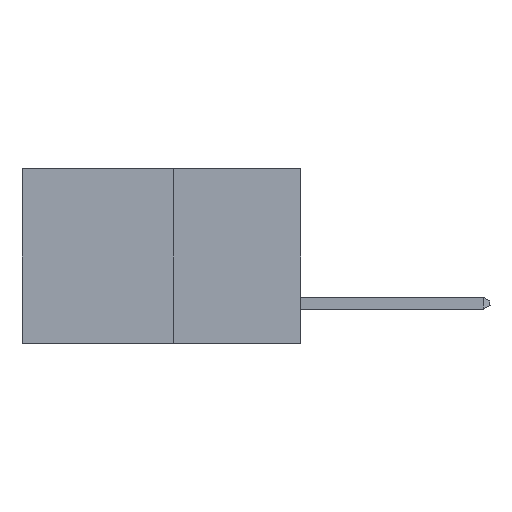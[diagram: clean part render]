
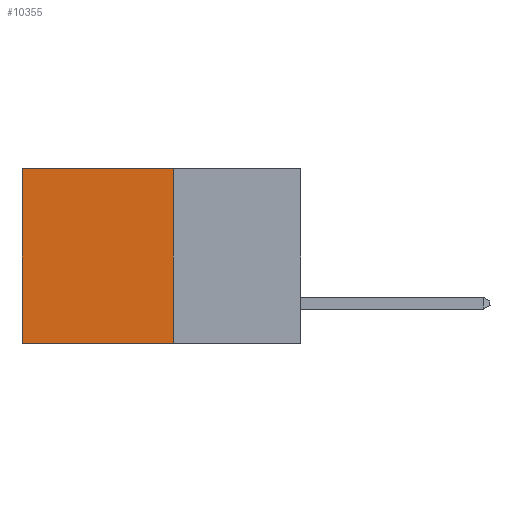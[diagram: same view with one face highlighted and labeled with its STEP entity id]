
A CAD part, left-side view. The second image highlights one B-rep face of the part: STEP entity #10355.
In plain terms, the highlighted planar face has unit normal (-1, 0, 0).
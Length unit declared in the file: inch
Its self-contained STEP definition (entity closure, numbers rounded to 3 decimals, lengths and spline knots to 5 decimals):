
#212 = VECTOR ( 'NONE', #16665, 39.37008 ) ;
#684 = ORIENTED_EDGE ( 'NONE', *, *, #13005, .F. ) ;
#1416 = LINE ( 'NONE', #24431, #15977 ) ;
#1437 = EDGE_CURVE ( 'NONE', #14065, #20318, #5223, .T. ) ;
#2071 = DIRECTION ( 'NONE',  ( 0., 0., -1. ) ) ;
#5223 = LINE ( 'NONE', #9895, #9431 ) ;
#5332 = CARTESIAN_POINT ( 'NONE',  ( 0.277, 0.59, -0.37 ) ) ;
#7688 = DIRECTION ( 'NONE',  ( 0., 0., -1. ) ) ;
#7889 = EDGE_CURVE ( 'NONE', #14002, #14274, #18704, .T. ) ;
#8149 = VECTOR ( 'NONE', #14058, 39.37008 ) ;
#8590 = CARTESIAN_POINT ( 'NONE',  ( 0.277, 0.59, 0. ) ) ;
#8659 = DIRECTION ( 'NONE',  ( 0., 1., 0. ) ) ;
#9170 = AXIS2_PLACEMENT_3D ( 'NONE', #23754, #13939, #2071 ) ;
#9354 = ORIENTED_EDGE ( 'NONE', *, *, #1437, .T. ) ;
#9431 = VECTOR ( 'NONE', #7688, 39.37008 ) ;
#9895 = CARTESIAN_POINT ( 'NONE',  ( 0.277, 0.59, -0.37 ) ) ;
#10355 = ADVANCED_FACE ( 'NONE', ( #16746 ), #21804, .F. ) ;
#12283 = EDGE_LOOP ( 'NONE', ( #9354, #684, #12313, #24118 ) ) ;
#12311 = CARTESIAN_POINT ( 'NONE',  ( 0.277, 0.27, 0. ) ) ;
#12313 = ORIENTED_EDGE ( 'NONE', *, *, #7889, .F. ) ;
#13005 = EDGE_CURVE ( 'NONE', #14274, #20318, #1416, .T. ) ;
#13184 = CARTESIAN_POINT ( 'NONE',  ( 0.277, 0.27, -0.37 ) ) ;
#13939 = DIRECTION ( 'NONE',  ( 1., 0., 0. ) ) ;
#14002 = VERTEX_POINT ( 'NONE', #12311 ) ;
#14058 = DIRECTION ( 'NONE',  ( 0., 0., -1. ) ) ;
#14065 = VERTEX_POINT ( 'NONE', #8590 ) ;
#14274 = VERTEX_POINT ( 'NONE', #13184 ) ;
#15451 = LINE ( 'NONE', #22607, #212 ) ;
#15977 = VECTOR ( 'NONE', #8659, 39.37008 ) ;
#16665 = DIRECTION ( 'NONE',  ( 0., 1., 0. ) ) ;
#16746 = FACE_OUTER_BOUND ( 'NONE', #12283, .T. ) ;
#17733 = EDGE_CURVE ( 'NONE', #14002, #14065, #15451, .T. ) ;
#18036 = CARTESIAN_POINT ( 'NONE',  ( 0.277, 0.27, -0.37 ) ) ;
#18704 = LINE ( 'NONE', #18036, #8149 ) ;
#20318 = VERTEX_POINT ( 'NONE', #5332 ) ;
#21804 = PLANE ( 'NONE',  #9170 ) ;
#22607 = CARTESIAN_POINT ( 'NONE',  ( 0.277, 0.27, 0. ) ) ;
#23754 = CARTESIAN_POINT ( 'NONE',  ( 0.277, 0.27, -0.37 ) ) ;
#24118 = ORIENTED_EDGE ( 'NONE', *, *, #17733, .T. ) ;
#24431 = CARTESIAN_POINT ( 'NONE',  ( 0.277, 0.27, -0.37 ) ) ;
